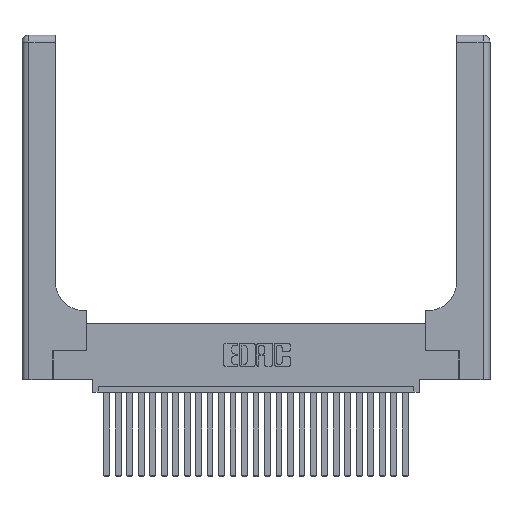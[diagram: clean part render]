
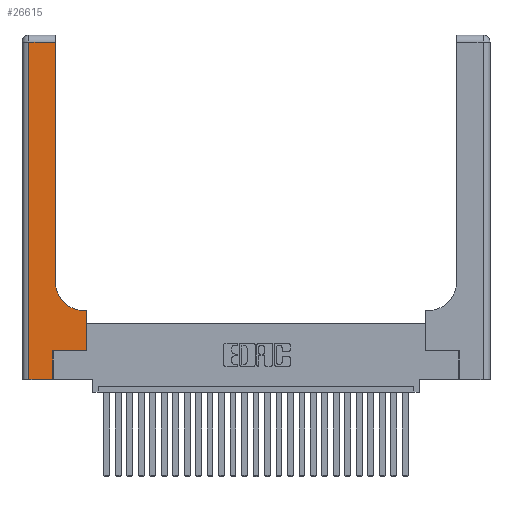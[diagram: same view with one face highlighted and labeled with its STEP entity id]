
A CAD part, top view. The second image highlights one B-rep face of the part: STEP entity #26615.
In plain terms, the highlighted planar face has unit normal (0, 0, 1).
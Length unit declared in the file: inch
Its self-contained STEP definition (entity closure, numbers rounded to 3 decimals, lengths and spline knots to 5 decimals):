
#790 = EDGE_CURVE ( 'NONE', #1051, #16335, #25471, .T. ) ;
#1051 = VERTEX_POINT ( 'NONE', #17861 ) ;
#1120 = EDGE_CURVE ( 'NONE', #14923, #25349, #11167, .T. ) ;
#1128 = ORIENTED_EDGE ( 'NONE', *, *, #18742, .T. ) ;
#1202 = VECTOR ( 'NONE', #25970, 39.37008 ) ;
#1205 = VECTOR ( 'NONE', #6775, 39.37008 ) ;
#1518 = LINE ( 'NONE', #25132, #14104 ) ;
#1994 = CARTESIAN_POINT ( 'NONE',  ( 0., 0., 0.37 ) ) ;
#2101 = CARTESIAN_POINT ( 'NONE',  ( 0.06, 3., 0.37 ) ) ;
#2653 = PLANE ( 'NONE',  #16385 ) ;
#3125 = VERTEX_POINT ( 'NONE', #27386 ) ;
#3369 = DIRECTION ( 'NONE',  ( 0., 0., -1. ) ) ;
#3419 = FACE_OUTER_BOUND ( 'NONE', #13431, .T. ) ;
#4583 = CARTESIAN_POINT ( 'NONE',  ( 0.269, 0., 0.37 ) ) ;
#4769 = DIRECTION ( 'NONE',  ( 1., 0., 0. ) ) ;
#5236 = ORIENTED_EDGE ( 'NONE', *, *, #790, .T. ) ;
#5255 = EDGE_CURVE ( 'NONE', #18415, #25972, #12057, .T. ) ;
#5322 = DIRECTION ( 'NONE',  ( -1., 0., 0. ) ) ;
#5494 = DIRECTION ( 'NONE',  ( 1., 0., 0. ) ) ;
#6000 = CARTESIAN_POINT ( 'NONE',  ( 0.5585, 0.6, 0.37 ) ) ;
#6122 = ORIENTED_EDGE ( 'NONE', *, *, #11003, .T. ) ;
#6775 = DIRECTION ( 'NONE',  ( -1., 0., 0. ) ) ;
#8262 = ORIENTED_EDGE ( 'NONE', *, *, #21193, .T. ) ;
#8672 = AXIS2_PLACEMENT_3D ( 'NONE', #18184, #3369, #5494 ) ;
#8929 = CARTESIAN_POINT ( 'NONE',  ( 0.2915, 0.6, 0.37 ) ) ;
#9057 = DIRECTION ( 'NONE',  ( 0., 0., -1. ) ) ;
#9346 = CARTESIAN_POINT ( 'NONE',  ( 0.06, 2.94, 0.37 ) ) ;
#9762 = ORIENTED_EDGE ( 'NONE', *, *, #18070, .T. ) ;
#9887 = LINE ( 'NONE', #2101, #24507 ) ;
#10308 = DIRECTION ( 'NONE',  ( 0., -1., 0. ) ) ;
#10721 = LINE ( 'NONE', #18391, #16661 ) ;
#11003 = EDGE_CURVE ( 'NONE', #16335, #23220, #19758, .T. ) ;
#11167 = LINE ( 'NONE', #1994, #19117 ) ;
#11258 = ORIENTED_EDGE ( 'NONE', *, *, #19910, .T. ) ;
#12057 = LINE ( 'NONE', #20227, #14693 ) ;
#12296 = DIRECTION ( 'NONE',  ( 0., 1., 0. ) ) ;
#12638 = DIRECTION ( 'NONE',  ( 1., 0., 0. ) ) ;
#12727 = ORIENTED_EDGE ( 'NONE', *, *, #5255, .T. ) ;
#13249 = VECTOR ( 'NONE', #4769, 39.37008 ) ;
#13431 = EDGE_LOOP ( 'NONE', ( #9762, #12727, #22948, #22437, #11258, #8262, #5236, #6122, #1128 ) ) ;
#14104 = VECTOR ( 'NONE', #25230, 39.37008 ) ;
#14693 = VECTOR ( 'NONE', #22734, 39.37008 ) ;
#14923 = VERTEX_POINT ( 'NONE', #23866 ) ;
#16335 = VERTEX_POINT ( 'NONE', #6000 ) ;
#16354 = CARTESIAN_POINT ( 'NONE',  ( 0.5415, 0.6, 0.37 ) ) ;
#16385 = AXIS2_PLACEMENT_3D ( 'NONE', #19597, #9057, #5322 ) ;
#16661 = VECTOR ( 'NONE', #12296, 39.37008 ) ;
#17534 = CARTESIAN_POINT ( 'NONE',  ( 0.2915, 2.94, 0.37 ) ) ;
#17861 = CARTESIAN_POINT ( 'NONE',  ( 0.5585, 0.25, 0.37 ) ) ;
#18070 = EDGE_CURVE ( 'NONE', #26326, #18415, #1518, .T. ) ;
#18184 = CARTESIAN_POINT ( 'NONE',  ( 0.5415, 0.85, 0.37 ) ) ;
#18391 = CARTESIAN_POINT ( 'NONE',  ( 0.269, 0., 0.37 ) ) ;
#18415 = VERTEX_POINT ( 'NONE', #17534 ) ;
#18742 = EDGE_CURVE ( 'NONE', #23220, #26326, #26046, .T. ) ;
#19117 = VECTOR ( 'NONE', #12638, 39.37008 ) ;
#19597 = CARTESIAN_POINT ( 'NONE',  ( 0., 3., 0.37 ) ) ;
#19758 = LINE ( 'NONE', #8929, #1205 ) ;
#19910 = EDGE_CURVE ( 'NONE', #25349, #3125, #10721, .T. ) ;
#20227 = CARTESIAN_POINT ( 'NONE',  ( 0., 2.94, 0.37 ) ) ;
#20645 = CARTESIAN_POINT ( 'NONE',  ( 0.2915, 0.85, 0.37 ) ) ;
#21193 = EDGE_CURVE ( 'NONE', #3125, #1051, #25261, .T. ) ;
#22437 = ORIENTED_EDGE ( 'NONE', *, *, #1120, .T. ) ;
#22562 = EDGE_CURVE ( 'NONE', #25972, #14923, #9887, .T. ) ;
#22734 = DIRECTION ( 'NONE',  ( -1., 0., 0. ) ) ;
#22948 = ORIENTED_EDGE ( 'NONE', *, *, #22562, .T. ) ;
#23220 = VERTEX_POINT ( 'NONE', #16354 ) ;
#23866 = CARTESIAN_POINT ( 'NONE',  ( 0.06, 0., 0.37 ) ) ;
#24507 = VECTOR ( 'NONE', #10308, 39.37008 ) ;
#25132 = CARTESIAN_POINT ( 'NONE',  ( 0.2915, 3., 0.37 ) ) ;
#25230 = DIRECTION ( 'NONE',  ( 0., 1., 0. ) ) ;
#25261 = LINE ( 'NONE', #25851, #13249 ) ;
#25349 = VERTEX_POINT ( 'NONE', #4583 ) ;
#25471 = LINE ( 'NONE', #26716, #1202 ) ;
#25851 = CARTESIAN_POINT ( 'NONE',  ( 0.269, 0.25, 0.37 ) ) ;
#25970 = DIRECTION ( 'NONE',  ( 0., 1., 0. ) ) ;
#25972 = VERTEX_POINT ( 'NONE', #9346 ) ;
#26046 = CIRCLE ( 'NONE', #8672, 0.25 ) ;
#26326 = VERTEX_POINT ( 'NONE', #20645 ) ;
#26615 = ADVANCED_FACE ( 'NONE', ( #3419 ), #2653, .F. ) ;
#26716 = CARTESIAN_POINT ( 'NONE',  ( 0.5585, 0.25, 0.37 ) ) ;
#27386 = CARTESIAN_POINT ( 'NONE',  ( 0.269, 0.25, 0.37 ) ) ;
